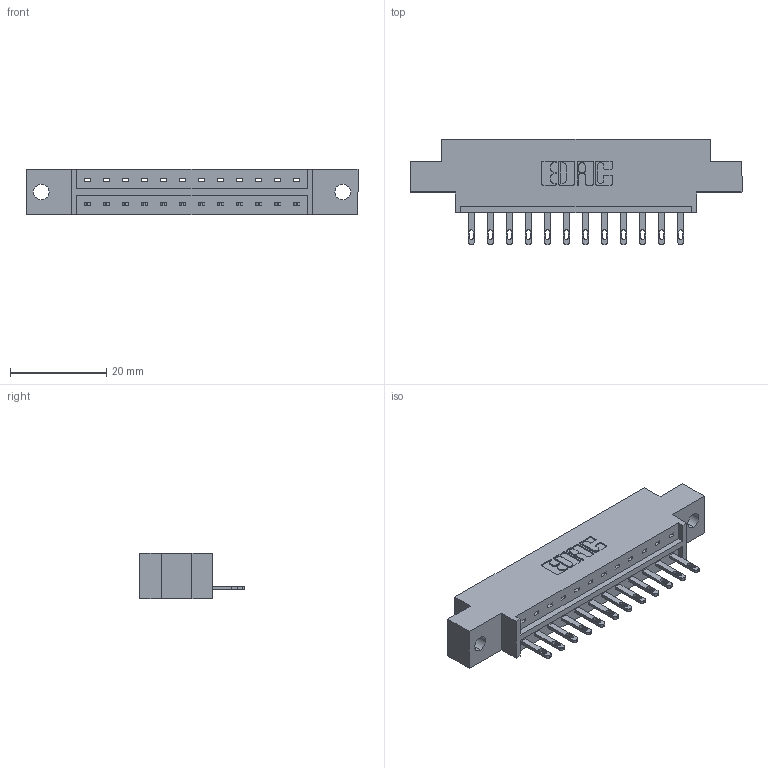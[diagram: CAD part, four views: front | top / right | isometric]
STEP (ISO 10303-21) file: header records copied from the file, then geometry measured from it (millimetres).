
FILE_DESCRIPTION (( 'STEP AP203' ), '1' );
FILE_NAME ('833-012-500-602.STEP', '2020-05-30T20:33:20', ( '' ), ( '' ), 'SwSTEP 2.0', 'SolidWorks 2020', '' );
FILE_SCHEMA (( 'CONFIG_CONTROL_DESIGN' ));
Length unit declared in the file: inch
Products named in the file (3): 833 Part_Offset - .128 Dia; 345-292-001_345-293-100; 833-012-500-602
Assembly tree (13 placements, depth 2):
  833-012-500-602
    833 Part_Offset - .128 Dia
    345-292-001_345-293-100  x12
Bounding box: 69.09 x 21.85 x 9.4 mm (x, y, z)
Volume: 6437.2 mm3; surface area: 6723.4 mm2
Topology: 13 solids, 13 shells, 766 faces, 2339 edges, 1558 vertices
Faces by surface type: plane 506, cylinder 260
Entity records: 11281 total; most frequent: CARTESIAN_POINT 1958, ORIENTED_EDGE 1906, DIRECTION 1713, EDGE_CURVE 953, VECTOR 821, LINE 821, VERTEX_POINT 634, AXIS2_PLACEMENT_3D 446
